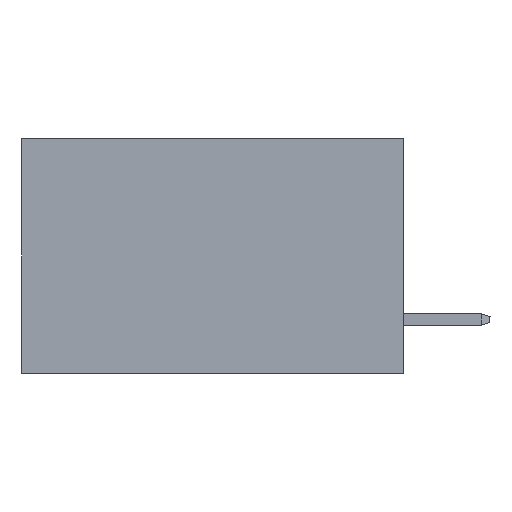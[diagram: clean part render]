
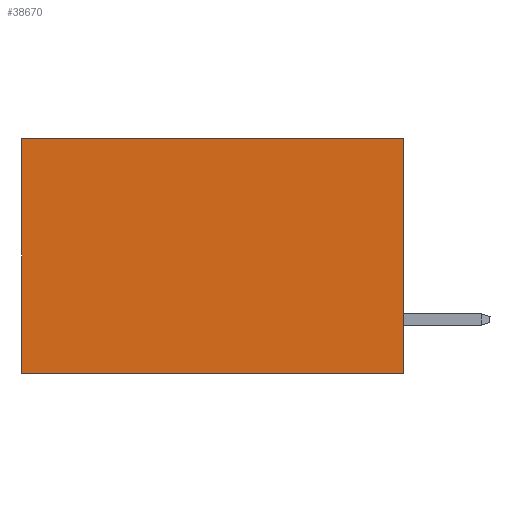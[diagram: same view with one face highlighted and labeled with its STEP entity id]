
A CAD part, left-side view. The second image highlights one B-rep face of the part: STEP entity #38670.
In plain terms, the highlighted planar face has unit normal (-1, 0, 0).
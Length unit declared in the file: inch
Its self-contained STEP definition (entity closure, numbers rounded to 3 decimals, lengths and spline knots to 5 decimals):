
#438 = CARTESIAN_POINT ( 'NONE',  ( 0.2875, 0., -0.37 ) ) ;
#3001 = CARTESIAN_POINT ( 'NONE',  ( 0.2875, 0., 0. ) ) ;
#3655 = VECTOR ( 'NONE', #16168, 39.37008 ) ;
#5565 = DIRECTION ( 'NONE',  ( 1., 0., 0. ) ) ;
#8365 = VERTEX_POINT ( 'NONE', #3001 ) ;
#8632 = ORIENTED_EDGE ( 'NONE', *, *, #25689, .T. ) ;
#9359 = VERTEX_POINT ( 'NONE', #21363 ) ;
#11587 = LINE ( 'NONE', #18559, #38299 ) ;
#12570 = CARTESIAN_POINT ( 'NONE',  ( 0.2875, 0., 0. ) ) ;
#15358 = EDGE_CURVE ( 'NONE', #8365, #31854, #27536, .T. ) ;
#15966 = EDGE_CURVE ( 'NONE', #34253, #9359, #11587, .T. ) ;
#16168 = DIRECTION ( 'NONE',  ( 0., 1., 0. ) ) ;
#17574 = LINE ( 'NONE', #31278, #37141 ) ;
#18559 = CARTESIAN_POINT ( 'NONE',  ( 0.2875, 0.6, 0. ) ) ;
#19893 = EDGE_LOOP ( 'NONE', ( #23734, #21743, #20931, #8632 ) ) ;
#20751 = CARTESIAN_POINT ( 'NONE',  ( 0.2875, 0., 0. ) ) ;
#20931 = ORIENTED_EDGE ( 'NONE', *, *, #15358, .F. ) ;
#21363 = CARTESIAN_POINT ( 'NONE',  ( 0.2875, 0.6, -0.37 ) ) ;
#21743 = ORIENTED_EDGE ( 'NONE', *, *, #22534, .F. ) ;
#21904 = DIRECTION ( 'NONE',  ( 0., 0., -1. ) ) ;
#22245 = LINE ( 'NONE', #12570, #3655 ) ;
#22534 = EDGE_CURVE ( 'NONE', #31854, #9359, #17574, .T. ) ;
#22629 = FACE_OUTER_BOUND ( 'NONE', #19893, .T. ) ;
#23734 = ORIENTED_EDGE ( 'NONE', *, *, #15966, .T. ) ;
#25689 = EDGE_CURVE ( 'NONE', #8365, #34253, #22245, .T. ) ;
#26239 = CARTESIAN_POINT ( 'NONE',  ( 0.2875, 0., 0. ) ) ;
#27536 = LINE ( 'NONE', #20751, #30364 ) ;
#30364 = VECTOR ( 'NONE', #34488, 39.37008 ) ;
#31278 = CARTESIAN_POINT ( 'NONE',  ( 0.2875, 0., -0.37 ) ) ;
#31333 = AXIS2_PLACEMENT_3D ( 'NONE', #26239, #5565, #32982 ) ;
#31790 = CARTESIAN_POINT ( 'NONE',  ( 0.2875, 0.6, 0. ) ) ;
#31854 = VERTEX_POINT ( 'NONE', #438 ) ;
#32982 = DIRECTION ( 'NONE',  ( 0., 0., -1. ) ) ;
#34253 = VERTEX_POINT ( 'NONE', #31790 ) ;
#34488 = DIRECTION ( 'NONE',  ( 0., 0., -1. ) ) ;
#36181 = DIRECTION ( 'NONE',  ( 0., 1., 0. ) ) ;
#36341 = PLANE ( 'NONE',  #31333 ) ;
#37141 = VECTOR ( 'NONE', #36181, 39.37008 ) ;
#38299 = VECTOR ( 'NONE', #21904, 39.37008 ) ;
#38670 = ADVANCED_FACE ( 'NONE', ( #22629 ), #36341, .F. ) ;
